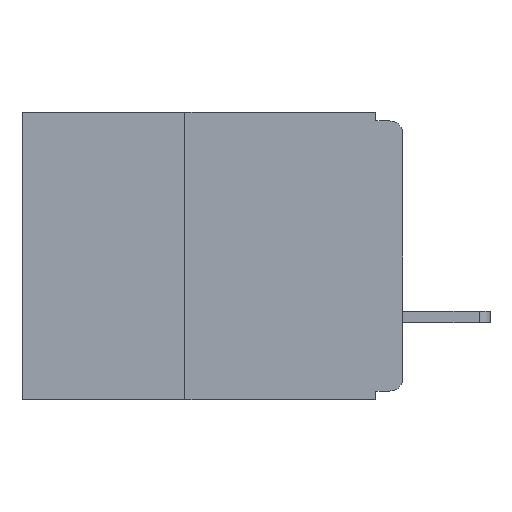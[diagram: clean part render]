
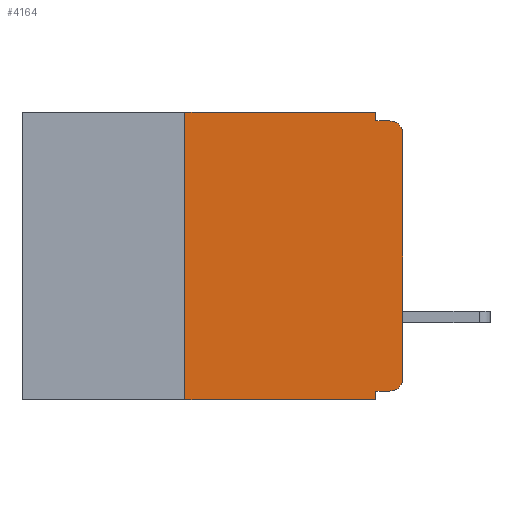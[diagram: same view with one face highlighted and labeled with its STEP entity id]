
A CAD part, left-side view. The second image highlights one B-rep face of the part: STEP entity #4164.
In plain terms, the highlighted planar face has unit normal (-1, 0, 0).
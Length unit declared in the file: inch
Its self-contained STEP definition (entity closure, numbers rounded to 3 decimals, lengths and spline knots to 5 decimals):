
#25 = VERTEX_POINT ( 'NONE', #8889 ) ;
#123 = CARTESIAN_POINT ( 'NONE',  ( 0., 0.437, 0. ) ) ;
#292 = VECTOR ( 'NONE', #15718, 39.37008 ) ;
#340 = ORIENTED_EDGE ( 'NONE', *, *, #1714, .F. ) ;
#391 = CARTESIAN_POINT ( 'NONE',  ( 0., 0.031, 0. ) ) ;
#425 = EDGE_CURVE ( 'NONE', #945, #14497, #10852, .T. ) ;
#532 = VERTEX_POINT ( 'NONE', #15994 ) ;
#554 = DIRECTION ( 'NONE',  ( 0., 0., 1. ) ) ;
#945 = VERTEX_POINT ( 'NONE', #5353 ) ;
#1277 = DIRECTION ( 'NONE',  ( 0., 0., 1. ) ) ;
#1714 = EDGE_CURVE ( 'NONE', #25, #1718, #2696, .T. ) ;
#1718 = VERTEX_POINT ( 'NONE', #391 ) ;
#1916 = ORIENTED_EDGE ( 'NONE', *, *, #425, .F. ) ;
#2288 = ORIENTED_EDGE ( 'NONE', *, *, #10231, .T. ) ;
#2311 = DIRECTION ( 'NONE',  ( 0., 0., -1. ) ) ;
#2696 = LINE ( 'NONE', #123, #15350 ) ;
#3053 = DIRECTION ( 'NONE',  ( 0., 0., -1. ) ) ;
#3124 = DIRECTION ( 'NONE',  ( 1., 0., 0. ) ) ;
#3249 = ORIENTED_EDGE ( 'NONE', *, *, #9696, .F. ) ;
#3265 = CARTESIAN_POINT ( 'NONE',  ( 0., 0.437, 0. ) ) ;
#3279 = PLANE ( 'NONE',  #6198 ) ;
#3552 = ORIENTED_EDGE ( 'NONE', *, *, #8290, .T. ) ;
#3627 = CARTESIAN_POINT ( 'NONE',  ( 0., 0., -0.305 ) ) ;
#4074 = CIRCLE ( 'NONE', #6160, 0.015 ) ;
#4100 = CARTESIAN_POINT ( 'NONE',  ( 0., 0., -0.01 ) ) ;
#4164 = ADVANCED_FACE ( 'NONE', ( #12965 ), #3279, .F. ) ;
#4588 = VERTEX_POINT ( 'NONE', #12193 ) ;
#4755 = DIRECTION ( 'NONE',  ( -1., 0., 0. ) ) ;
#4792 = LINE ( 'NONE', #15051, #11097 ) ;
#4832 = CARTESIAN_POINT ( 'NONE',  ( 0., 0.031, 0. ) ) ;
#5346 = DIRECTION ( 'NONE',  ( 0., -1., 0. ) ) ;
#5353 = CARTESIAN_POINT ( 'NONE',  ( 0., 0.031, -0.32 ) ) ;
#5401 = ORIENTED_EDGE ( 'NONE', *, *, #15226, .F. ) ;
#5563 = VERTEX_POINT ( 'NONE', #11808 ) ;
#5759 = CARTESIAN_POINT ( 'NONE',  ( 0., 0., 0. ) ) ;
#5763 = DIRECTION ( 'NONE',  ( -1., 0., 0. ) ) ;
#5832 = CIRCLE ( 'NONE', #12797, 0.015 ) ;
#5909 = ORIENTED_EDGE ( 'NONE', *, *, #15385, .F. ) ;
#5986 = VECTOR ( 'NONE', #1277, 39.37008 ) ;
#6160 = AXIS2_PLACEMENT_3D ( 'NONE', #13164, #5763, #14292 ) ;
#6198 = AXIS2_PLACEMENT_3D ( 'NONE', #3265, #3124, #3053 ) ;
#6387 = LINE ( 'NONE', #10273, #5986 ) ;
#7176 = ORIENTED_EDGE ( 'NONE', *, *, #10124, .T. ) ;
#7521 = VECTOR ( 'NONE', #8042, 39.37008 ) ;
#7602 = ORIENTED_EDGE ( 'NONE', *, *, #15463, .T. ) ;
#7676 = LINE ( 'NONE', #5759, #10631 ) ;
#7779 = VECTOR ( 'NONE', #2311, 39.37008 ) ;
#8042 = DIRECTION ( 'NONE',  ( 0., 0., -1. ) ) ;
#8090 = LINE ( 'NONE', #4100, #10976 ) ;
#8290 = EDGE_CURVE ( 'NONE', #10656, #4588, #7676, .T. ) ;
#8561 = CARTESIAN_POINT ( 'NONE',  ( 0., 0.031, -0.33 ) ) ;
#8580 = CARTESIAN_POINT ( 'NONE',  ( 0., 0.25, -0.33 ) ) ;
#8728 = EDGE_CURVE ( 'NONE', #532, #11187, #8090, .T. ) ;
#8889 = CARTESIAN_POINT ( 'NONE',  ( 0., 0.25, 0. ) ) ;
#9696 = EDGE_CURVE ( 'NONE', #5563, #945, #10953, .T. ) ;
#10103 = DIRECTION ( 'NONE',  ( 0., -1., 0. ) ) ;
#10124 = EDGE_CURVE ( 'NONE', #4588, #11187, #4074, .T. ) ;
#10231 = EDGE_CURVE ( 'NONE', #5563, #10656, #5832, .T. ) ;
#10273 = CARTESIAN_POINT ( 'NONE',  ( 0., 0.25, -0.33 ) ) ;
#10631 = VECTOR ( 'NONE', #554, 39.37008 ) ;
#10656 = VERTEX_POINT ( 'NONE', #3627 ) ;
#10852 = LINE ( 'NONE', #8561, #7521 ) ;
#10953 = LINE ( 'NONE', #11160, #292 ) ;
#10976 = VECTOR ( 'NONE', #5346, 39.37008 ) ;
#11097 = VECTOR ( 'NONE', #11565, 39.37008 ) ;
#11160 = CARTESIAN_POINT ( 'NONE',  ( 0., 0., -0.32 ) ) ;
#11187 = VERTEX_POINT ( 'NONE', #14496 ) ;
#11565 = DIRECTION ( 'NONE',  ( 0., -1., 0. ) ) ;
#11788 = EDGE_LOOP ( 'NONE', ( #3552, #7176, #14811, #5401, #340, #5909, #7602, #1916, #3249, #2288 ) ) ;
#11808 = CARTESIAN_POINT ( 'NONE',  ( 0., 0.015, -0.32 ) ) ;
#12193 = CARTESIAN_POINT ( 'NONE',  ( 0., 0., -0.025 ) ) ;
#12215 = CARTESIAN_POINT ( 'NONE',  ( 0., 0.015, -0.305 ) ) ;
#12797 = AXIS2_PLACEMENT_3D ( 'NONE', #12215, #4755, #13393 ) ;
#12965 = FACE_OUTER_BOUND ( 'NONE', #11788, .T. ) ;
#13164 = CARTESIAN_POINT ( 'NONE',  ( 0., 0.015, -0.025 ) ) ;
#13393 = DIRECTION ( 'NONE',  ( 0., 0., -1. ) ) ;
#13432 = CARTESIAN_POINT ( 'NONE',  ( 0., 0.031, -0.33 ) ) ;
#13832 = VERTEX_POINT ( 'NONE', #8580 ) ;
#14183 = LINE ( 'NONE', #4832, #7779 ) ;
#14292 = DIRECTION ( 'NONE',  ( 0., 0., -1. ) ) ;
#14496 = CARTESIAN_POINT ( 'NONE',  ( 0., 0.015, -0.01 ) ) ;
#14497 = VERTEX_POINT ( 'NONE', #13432 ) ;
#14811 = ORIENTED_EDGE ( 'NONE', *, *, #8728, .F. ) ;
#15051 = CARTESIAN_POINT ( 'NONE',  ( 0., 0.437, -0.33 ) ) ;
#15226 = EDGE_CURVE ( 'NONE', #1718, #532, #14183, .T. ) ;
#15350 = VECTOR ( 'NONE', #10103, 39.37008 ) ;
#15385 = EDGE_CURVE ( 'NONE', #13832, #25, #6387, .T. ) ;
#15463 = EDGE_CURVE ( 'NONE', #13832, #14497, #4792, .T. ) ;
#15718 = DIRECTION ( 'NONE',  ( 0., 1., 0. ) ) ;
#15994 = CARTESIAN_POINT ( 'NONE',  ( 0., 0.031, -0.01 ) ) ;
